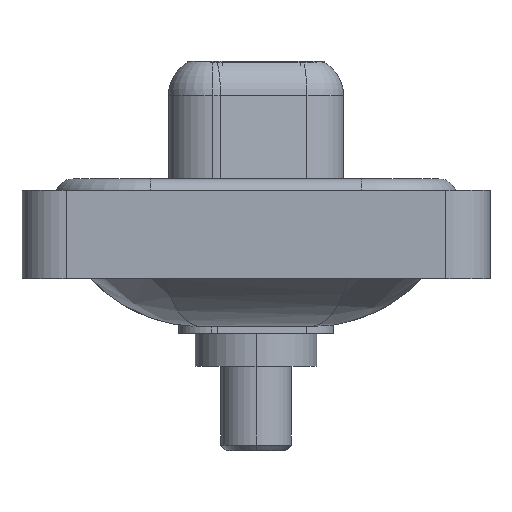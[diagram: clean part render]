
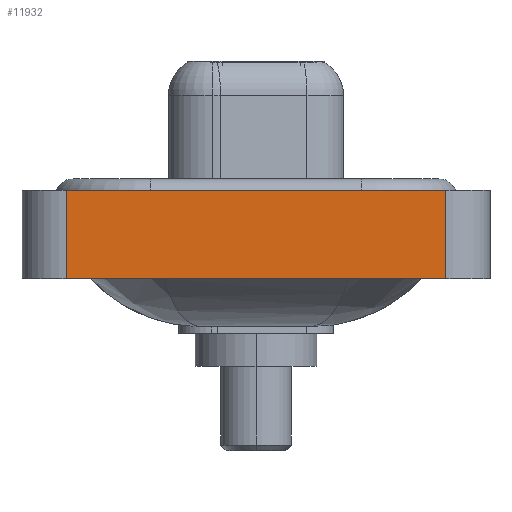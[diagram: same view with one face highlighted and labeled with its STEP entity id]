
A CAD part, left-side view. The second image highlights one B-rep face of the part: STEP entity #11932.
In plain terms, the highlighted planar face has unit normal (-1, 0, 0).
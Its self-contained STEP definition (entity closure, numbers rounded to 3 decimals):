
#86 = CARTESIAN_POINT ( 'NONE',  ( -7.25, 8.55, -3.6 ) ) ;
#1211 = CARTESIAN_POINT ( 'NONE',  ( -7.25, -8.55, -3.6 ) ) ;
#1379 = AXIS2_PLACEMENT_3D ( 'NONE', #11985, #12147, #8138 ) ;
#1410 = PLANE ( 'NONE',  #1379 ) ;
#2339 = LINE ( 'NONE', #7410, #3120 ) ;
#2602 = CARTESIAN_POINT ( 'NONE',  ( -7.25, 8.55, 0.4 ) ) ;
#2880 = FACE_OUTER_BOUND ( 'NONE', #4430, .T. ) ;
#2885 = EDGE_CURVE ( 'NONE', #15758, #6568, #2339, .T. ) ;
#3120 = VECTOR ( 'NONE', #10080, 1000. ) ;
#3306 = ORIENTED_EDGE ( 'NONE', *, *, #5400, .F. ) ;
#3496 = DIRECTION ( 'NONE',  ( 0., 0., 1. ) ) ;
#3816 = LINE ( 'NONE', #1211, #15305 ) ;
#4430 = EDGE_LOOP ( 'NONE', ( #13820, #9429, #3306, #10742 ) ) ;
#4999 = VECTOR ( 'NONE', #3496, 1000. ) ;
#5127 = DIRECTION ( 'NONE',  ( 0., -1., 0. ) ) ;
#5400 = EDGE_CURVE ( 'NONE', #14880, #15758, #11375, .T. ) ;
#6568 = VERTEX_POINT ( 'NONE', #7533 ) ;
#7410 = CARTESIAN_POINT ( 'NONE',  ( -7.25, -8.55, 0.4 ) ) ;
#7533 = CARTESIAN_POINT ( 'NONE',  ( -7.25, -8.55, 0.4 ) ) ;
#7567 = VERTEX_POINT ( 'NONE', #13232 ) ;
#8138 = DIRECTION ( 'NONE',  ( 0., 0., 1. ) ) ;
#9350 = VECTOR ( 'NONE', #5127, 1000. ) ;
#9429 = ORIENTED_EDGE ( 'NONE', *, *, #2885, .F. ) ;
#10080 = DIRECTION ( 'NONE',  ( 0., -1., 0. ) ) ;
#10742 = ORIENTED_EDGE ( 'NONE', *, *, #11902, .T. ) ;
#11293 = CARTESIAN_POINT ( 'NONE',  ( -7.25, 8.55, -3.6 ) ) ;
#11375 = LINE ( 'NONE', #11293, #4999 ) ;
#11637 = LINE ( 'NONE', #16829, #9350 ) ;
#11902 = EDGE_CURVE ( 'NONE', #14880, #7567, #11637, .T. ) ;
#11932 = ADVANCED_FACE ( 'NONE', ( #2880 ), #1410, .T. ) ;
#11985 = CARTESIAN_POINT ( 'NONE',  ( -7.25, -8.55, -3.6 ) ) ;
#12147 = DIRECTION ( 'NONE',  ( -1., 0., 0. ) ) ;
#13232 = CARTESIAN_POINT ( 'NONE',  ( -7.25, -8.55, -3.6 ) ) ;
#13820 = ORIENTED_EDGE ( 'NONE', *, *, #16069, .T. ) ;
#14880 = VERTEX_POINT ( 'NONE', #86 ) ;
#15305 = VECTOR ( 'NONE', #16894, 1000. ) ;
#15758 = VERTEX_POINT ( 'NONE', #2602 ) ;
#16069 = EDGE_CURVE ( 'NONE', #7567, #6568, #3816, .T. ) ;
#16829 = CARTESIAN_POINT ( 'NONE',  ( -7.25, -8.55, -3.6 ) ) ;
#16894 = DIRECTION ( 'NONE',  ( 0., 0., 1. ) ) ;
